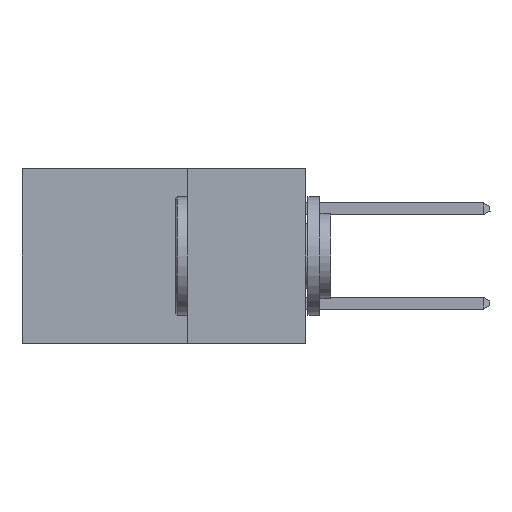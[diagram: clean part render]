
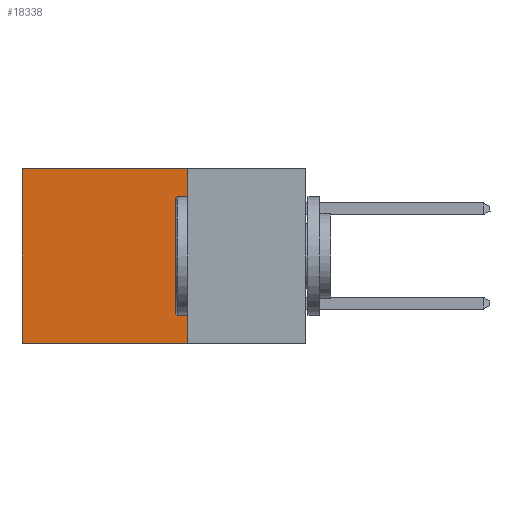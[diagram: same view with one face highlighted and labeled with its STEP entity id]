
A CAD part, left-side view. The second image highlights one B-rep face of the part: STEP entity #18338.
In plain terms, the highlighted planar face has unit normal (-1, 0, 0).
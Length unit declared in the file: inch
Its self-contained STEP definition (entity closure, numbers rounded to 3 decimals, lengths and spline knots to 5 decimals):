
#866 = VECTOR ( 'NONE', #26207, 39.37008 ) ;
#1712 = DIRECTION ( 'NONE',  ( 0., 1., 0. ) ) ;
#2613 = CARTESIAN_POINT ( 'NONE',  ( 0.298, 0.6, -0.37 ) ) ;
#3602 = VERTEX_POINT ( 'NONE', #20888 ) ;
#3702 = FACE_OUTER_BOUND ( 'NONE', #7963, .T. ) ;
#5233 = DIRECTION ( 'NONE',  ( 0., 0., -1. ) ) ;
#6308 = VERTEX_POINT ( 'NONE', #16816 ) ;
#7195 = VERTEX_POINT ( 'NONE', #14900 ) ;
#7596 = LINE ( 'NONE', #10792, #866 ) ;
#7952 = CARTESIAN_POINT ( 'NONE',  ( 0.298, 0.25, 0. ) ) ;
#7963 = EDGE_LOOP ( 'NONE', ( #18865, #10094, #30997, #11931 ) ) ;
#8669 = AXIS2_PLACEMENT_3D ( 'NONE', #17107, #14352, #19707 ) ;
#10094 = ORIENTED_EDGE ( 'NONE', *, *, #13122, .F. ) ;
#10410 = DIRECTION ( 'NONE',  ( 0., 0., -1. ) ) ;
#10755 = VECTOR ( 'NONE', #10410, 39.37008 ) ;
#10792 = CARTESIAN_POINT ( 'NONE',  ( 0.298, 0.25, -0.37 ) ) ;
#11856 = EDGE_CURVE ( 'NONE', #6308, #16490, #18257, .T. ) ;
#11931 = ORIENTED_EDGE ( 'NONE', *, *, #21792, .T. ) ;
#12961 = CARTESIAN_POINT ( 'NONE',  ( 0.298, 0.6, 0. ) ) ;
#13122 = EDGE_CURVE ( 'NONE', #7195, #16490, #7596, .T. ) ;
#13959 = LINE ( 'NONE', #32160, #21802 ) ;
#14352 = DIRECTION ( 'NONE',  ( 1., 0., 0. ) ) ;
#14900 = CARTESIAN_POINT ( 'NONE',  ( 0.298, 0.25, -0.37 ) ) ;
#16490 = VERTEX_POINT ( 'NONE', #2613 ) ;
#16816 = CARTESIAN_POINT ( 'NONE',  ( 0.298, 0.6, 0. ) ) ;
#16901 = PLANE ( 'NONE',  #8669 ) ;
#17107 = CARTESIAN_POINT ( 'NONE',  ( 0.298, 0.25, 0. ) ) ;
#17196 = VECTOR ( 'NONE', #5233, 39.37008 ) ;
#18257 = LINE ( 'NONE', #12961, #10755 ) ;
#18338 = ADVANCED_FACE ( 'NONE', ( #3702 ), #16901, .F. ) ;
#18865 = ORIENTED_EDGE ( 'NONE', *, *, #11856, .T. ) ;
#19707 = DIRECTION ( 'NONE',  ( 0., 0., -1. ) ) ;
#20888 = CARTESIAN_POINT ( 'NONE',  ( 0.298, 0.25, 0. ) ) ;
#21792 = EDGE_CURVE ( 'NONE', #3602, #6308, #13959, .T. ) ;
#21802 = VECTOR ( 'NONE', #1712, 39.37008 ) ;
#26207 = DIRECTION ( 'NONE',  ( 0., 1., 0. ) ) ;
#28246 = LINE ( 'NONE', #7952, #17196 ) ;
#30871 = EDGE_CURVE ( 'NONE', #3602, #7195, #28246, .T. ) ;
#30997 = ORIENTED_EDGE ( 'NONE', *, *, #30871, .F. ) ;
#32160 = CARTESIAN_POINT ( 'NONE',  ( 0.298, 0.25, 0. ) ) ;
